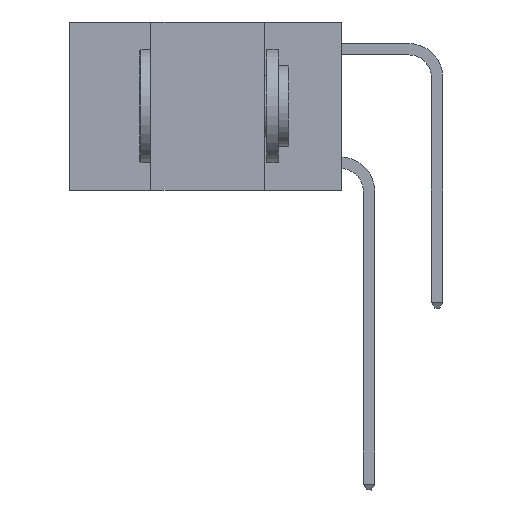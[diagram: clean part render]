
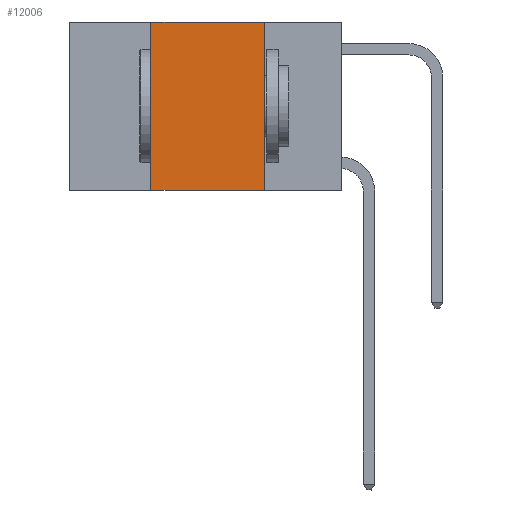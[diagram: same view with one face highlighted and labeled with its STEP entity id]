
A CAD part, left-side view. The second image highlights one B-rep face of the part: STEP entity #12006.
In plain terms, the highlighted planar face has unit normal (-1, 0, 0).
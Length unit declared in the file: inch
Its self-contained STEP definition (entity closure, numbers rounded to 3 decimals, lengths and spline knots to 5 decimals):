
#147 = PLANE ( 'NONE',  #5115 ) ;
#329 = VERTEX_POINT ( 'NONE', #17651 ) ;
#652 = LINE ( 'NONE', #6303, #16353 ) ;
#800 = EDGE_CURVE ( 'NONE', #5613, #329, #652, .T. ) ;
#1126 = ORIENTED_EDGE ( 'NONE', *, *, #10888, .F. ) ;
#1702 = DIRECTION ( 'NONE',  ( 0., 0., -1. ) ) ;
#1760 = EDGE_CURVE ( 'NONE', #5613, #17410, #16588, .T. ) ;
#2248 = CARTESIAN_POINT ( 'NONE',  ( 0., 0.17, 0. ) ) ;
#2365 = VECTOR ( 'NONE', #17318, 39.37008 ) ;
#3063 = ORIENTED_EDGE ( 'NONE', *, *, #800, .F. ) ;
#4513 = CARTESIAN_POINT ( 'NONE',  ( 0., 0.6, -0.37 ) ) ;
#5115 = AXIS2_PLACEMENT_3D ( 'NONE', #9316, #10824, #1702 ) ;
#5213 = CARTESIAN_POINT ( 'NONE',  ( 0., 0.6, 0. ) ) ;
#5613 = VERTEX_POINT ( 'NONE', #14447 ) ;
#6303 = CARTESIAN_POINT ( 'NONE',  ( 0., 0.42, 0. ) ) ;
#6625 = ORIENTED_EDGE ( 'NONE', *, *, #1760, .T. ) ;
#7883 = CARTESIAN_POINT ( 'NONE',  ( 0., 0.17, 0. ) ) ;
#8982 = LINE ( 'NONE', #2248, #12483 ) ;
#9007 = EDGE_LOOP ( 'NONE', ( #13007, #1126, #3063, #6625 ) ) ;
#9105 = CARTESIAN_POINT ( 'NONE',  ( 0., 0.17, -0.37 ) ) ;
#9316 = CARTESIAN_POINT ( 'NONE',  ( 0., 0.6, 0. ) ) ;
#10824 = DIRECTION ( 'NONE',  ( 1., 0., 0. ) ) ;
#10888 = EDGE_CURVE ( 'NONE', #329, #15878, #18457, .T. ) ;
#11491 = DIRECTION ( 'NONE',  ( 0., 0., 1. ) ) ;
#12006 = ADVANCED_FACE ( 'NONE', ( #14648 ), #147, .F. ) ;
#12483 = VECTOR ( 'NONE', #12836, 39.37008 ) ;
#12530 = VECTOR ( 'NONE', #19647, 39.37008 ) ;
#12836 = DIRECTION ( 'NONE',  ( 0., 0., -1. ) ) ;
#13007 = ORIENTED_EDGE ( 'NONE', *, *, #19084, .F. ) ;
#14447 = CARTESIAN_POINT ( 'NONE',  ( 0., 0.42, -0.37 ) ) ;
#14648 = FACE_OUTER_BOUND ( 'NONE', #9007, .T. ) ;
#15878 = VERTEX_POINT ( 'NONE', #7883 ) ;
#16353 = VECTOR ( 'NONE', #11491, 39.37008 ) ;
#16588 = LINE ( 'NONE', #4513, #12530 ) ;
#17318 = DIRECTION ( 'NONE',  ( 0., -1., 0. ) ) ;
#17410 = VERTEX_POINT ( 'NONE', #9105 ) ;
#17651 = CARTESIAN_POINT ( 'NONE',  ( 0., 0.42, 0. ) ) ;
#18457 = LINE ( 'NONE', #5213, #2365 ) ;
#19084 = EDGE_CURVE ( 'NONE', #15878, #17410, #8982, .T. ) ;
#19647 = DIRECTION ( 'NONE',  ( 0., -1., 0. ) ) ;
